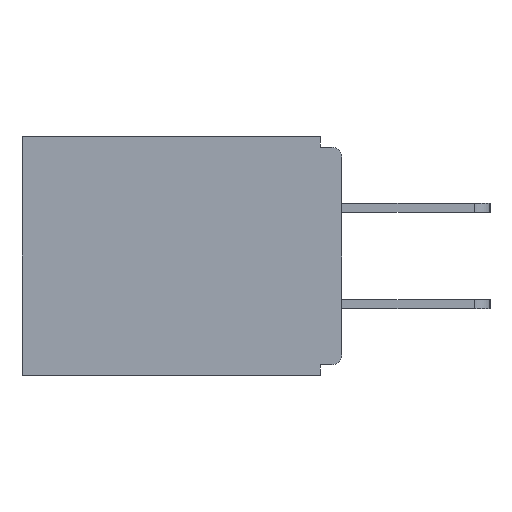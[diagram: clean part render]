
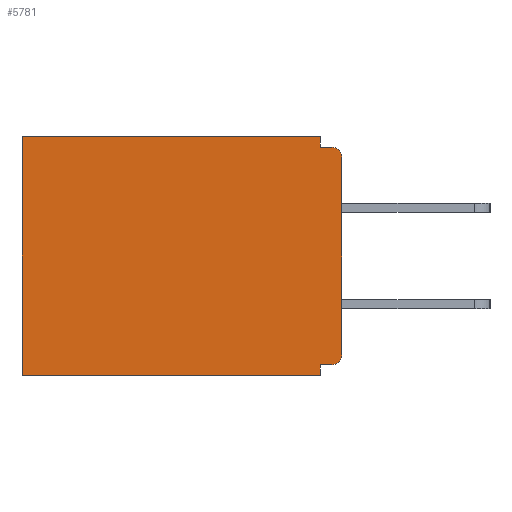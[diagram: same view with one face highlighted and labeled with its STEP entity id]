
A CAD part, left-side view. The second image highlights one B-rep face of the part: STEP entity #5781.
In plain terms, the highlighted planar face has unit normal (-1, 0, 0).
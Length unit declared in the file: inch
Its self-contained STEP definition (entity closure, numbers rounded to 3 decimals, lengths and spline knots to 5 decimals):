
#354 = ORIENTED_EDGE ( 'NONE', *, *, #15700, .T. ) ;
#453 = EDGE_LOOP ( 'NONE', ( #9938, #13341, #6482, #354, #15144, #15470, #15847, #8281, #16747, #697 ) ) ;
#524 = VECTOR ( 'NONE', #3283, 39.37008 ) ;
#613 = DIRECTION ( 'NONE',  ( 0., -1., 0. ) ) ;
#697 = ORIENTED_EDGE ( 'NONE', *, *, #2423, .F. ) ;
#909 = LINE ( 'NONE', #3505, #4386 ) ;
#920 = CARTESIAN_POINT ( 'NONE',  ( 0.298, 0., 0. ) ) ;
#976 = CARTESIAN_POINT ( 'NONE',  ( 0.298, 0.031, -0.343 ) ) ;
#1098 = CARTESIAN_POINT ( 'NONE',  ( 0.298, 0.031, -0.343 ) ) ;
#1258 = DIRECTION ( 'NONE',  ( 0., 0., -1. ) ) ;
#1315 = DIRECTION ( 'NONE',  ( 0., 0., -1. ) ) ;
#1338 = LINE ( 'NONE', #15859, #11560 ) ;
#1551 = VERTEX_POINT ( 'NONE', #4776 ) ;
#2003 = EDGE_CURVE ( 'NONE', #15779, #13485, #1338, .T. ) ;
#2386 = EDGE_CURVE ( 'NONE', #1551, #13485, #9853, .T. ) ;
#2416 = DIRECTION ( 'NONE',  ( 0., 0., -1. ) ) ;
#2423 = EDGE_CURVE ( 'NONE', #2425, #16293, #11118, .T. ) ;
#2425 = VERTEX_POINT ( 'NONE', #15505 ) ;
#3283 = DIRECTION ( 'NONE',  ( 0., 1., 0. ) ) ;
#3327 = CARTESIAN_POINT ( 'NONE',  ( 0.298, 0.031, -0.015 ) ) ;
#3401 = CARTESIAN_POINT ( 'NONE',  ( 0.298, 0.46, 0. ) ) ;
#3505 = CARTESIAN_POINT ( 'NONE',  ( 0.298, 0., 0. ) ) ;
#3656 = DIRECTION ( 'NONE',  ( 1., 0., 0. ) ) ;
#3689 = LINE ( 'NONE', #1098, #13922 ) ;
#4386 = VECTOR ( 'NONE', #8826, 39.37008 ) ;
#4726 = CARTESIAN_POINT ( 'NONE',  ( 0.298, 0., -0.015 ) ) ;
#4776 = CARTESIAN_POINT ( 'NONE',  ( 0.298, 0.46, 0. ) ) ;
#4787 = VERTEX_POINT ( 'NONE', #5956 ) ;
#5124 = DIRECTION ( 'NONE',  ( 0., 0., -1. ) ) ;
#5208 = DIRECTION ( 'NONE',  ( -1., 0., 0. ) ) ;
#5724 = DIRECTION ( 'NONE',  ( 0., 0., -1. ) ) ;
#5781 = ADVANCED_FACE ( 'NONE', ( #6242 ), #6422, .F. ) ;
#5787 = CARTESIAN_POINT ( 'NONE',  ( 0.298, 0.031, -0.328 ) ) ;
#5956 = CARTESIAN_POINT ( 'NONE',  ( 0.298, 0.015, -0.015 ) ) ;
#6127 = AXIS2_PLACEMENT_3D ( 'NONE', #10702, #5208, #1315 ) ;
#6157 = DIRECTION ( 'NONE',  ( 0., 0., -1. ) ) ;
#6242 = FACE_OUTER_BOUND ( 'NONE', #453, .T. ) ;
#6422 = PLANE ( 'NONE',  #11813 ) ;
#6482 = ORIENTED_EDGE ( 'NONE', *, *, #17139, .F. ) ;
#7143 = VECTOR ( 'NONE', #6157, 39.37008 ) ;
#7389 = CARTESIAN_POINT ( 'NONE',  ( 0.298, 0., -0.328 ) ) ;
#8281 = ORIENTED_EDGE ( 'NONE', *, *, #15539, .F. ) ;
#8791 = VERTEX_POINT ( 'NONE', #3327 ) ;
#8826 = DIRECTION ( 'NONE',  ( 0., 1., 0. ) ) ;
#9853 = LINE ( 'NONE', #3401, #10479 ) ;
#9938 = ORIENTED_EDGE ( 'NONE', *, *, #16490, .T. ) ;
#10378 = CARTESIAN_POINT ( 'NONE',  ( 0.298, 0.46, -0.343 ) ) ;
#10451 = CARTESIAN_POINT ( 'NONE',  ( 0.298, 0.015, -0.328 ) ) ;
#10479 = VECTOR ( 'NONE', #12714, 39.37008 ) ;
#10702 = CARTESIAN_POINT ( 'NONE',  ( 0.298, 0.015, -0.313 ) ) ;
#10986 = LINE ( 'NONE', #11992, #16833 ) ;
#11118 = LINE ( 'NONE', #920, #7143 ) ;
#11171 = EDGE_CURVE ( 'NONE', #14569, #16293, #12277, .T. ) ;
#11560 = VECTOR ( 'NONE', #12066, 39.37008 ) ;
#11813 = AXIS2_PLACEMENT_3D ( 'NONE', #15782, #3656, #1258 ) ;
#11929 = EDGE_CURVE ( 'NONE', #8791, #4787, #15597, .T. ) ;
#11992 = CARTESIAN_POINT ( 'NONE',  ( 0.298, 0.031, -0.343 ) ) ;
#12066 = DIRECTION ( 'NONE',  ( 0., 1., 0. ) ) ;
#12277 = CIRCLE ( 'NONE', #6127, 0.015 ) ;
#12663 = VERTEX_POINT ( 'NONE', #13480 ) ;
#12714 = DIRECTION ( 'NONE',  ( 0., 0., -1. ) ) ;
#12969 = LINE ( 'NONE', #7389, #524 ) ;
#13250 = DIRECTION ( 'NONE',  ( -1., 0., 0. ) ) ;
#13341 = ORIENTED_EDGE ( 'NONE', *, *, #11929, .F. ) ;
#13480 = CARTESIAN_POINT ( 'NONE',  ( 0.298, 0.031, 0. ) ) ;
#13485 = VERTEX_POINT ( 'NONE', #10378 ) ;
#13922 = VECTOR ( 'NONE', #2416, 39.37008 ) ;
#14086 = VERTEX_POINT ( 'NONE', #5787 ) ;
#14138 = CIRCLE ( 'NONE', #14456, 0.015 ) ;
#14456 = AXIS2_PLACEMENT_3D ( 'NONE', #14631, #13250, #5124 ) ;
#14569 = VERTEX_POINT ( 'NONE', #10451 ) ;
#14631 = CARTESIAN_POINT ( 'NONE',  ( 0.298, 0.015, -0.03 ) ) ;
#14710 = CARTESIAN_POINT ( 'NONE',  ( 0.298, 0., -0.313 ) ) ;
#15144 = ORIENTED_EDGE ( 'NONE', *, *, #2386, .T. ) ;
#15383 = VECTOR ( 'NONE', #613, 39.37008 ) ;
#15470 = ORIENTED_EDGE ( 'NONE', *, *, #2003, .F. ) ;
#15505 = CARTESIAN_POINT ( 'NONE',  ( 0.298, 0., -0.03 ) ) ;
#15539 = EDGE_CURVE ( 'NONE', #14569, #14086, #12969, .T. ) ;
#15597 = LINE ( 'NONE', #4726, #15383 ) ;
#15700 = EDGE_CURVE ( 'NONE', #12663, #1551, #909, .T. ) ;
#15779 = VERTEX_POINT ( 'NONE', #976 ) ;
#15782 = CARTESIAN_POINT ( 'NONE',  ( 0.298, 0., 0. ) ) ;
#15847 = ORIENTED_EDGE ( 'NONE', *, *, #17089, .F. ) ;
#15859 = CARTESIAN_POINT ( 'NONE',  ( 0.298, 0., -0.343 ) ) ;
#16293 = VERTEX_POINT ( 'NONE', #14710 ) ;
#16490 = EDGE_CURVE ( 'NONE', #2425, #4787, #14138, .T. ) ;
#16747 = ORIENTED_EDGE ( 'NONE', *, *, #11171, .T. ) ;
#16833 = VECTOR ( 'NONE', #5724, 39.37008 ) ;
#17089 = EDGE_CURVE ( 'NONE', #14086, #15779, #3689, .T. ) ;
#17139 = EDGE_CURVE ( 'NONE', #12663, #8791, #10986, .T. ) ;
